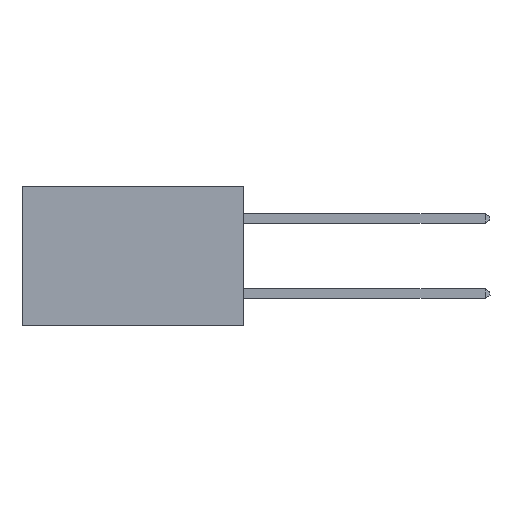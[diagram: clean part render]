
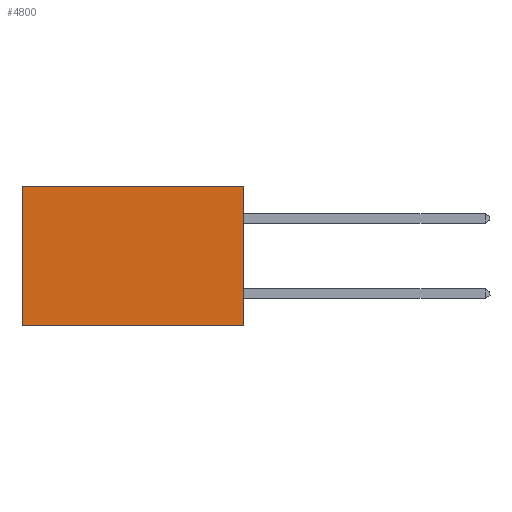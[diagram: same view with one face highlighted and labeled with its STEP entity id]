
A CAD part, left-side view. The second image highlights one B-rep face of the part: STEP entity #4800.
In plain terms, the highlighted planar face has unit normal (-1, 0, 0).
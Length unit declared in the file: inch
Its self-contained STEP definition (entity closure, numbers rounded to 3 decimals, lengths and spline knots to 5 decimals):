
#14 = FACE_OUTER_BOUND ( 'NONE', #2505, .T. ) ;
#333 = ORIENTED_EDGE ( 'NONE', *, *, #8557, .F. ) ;
#865 = EDGE_CURVE ( 'NONE', #5852, #4934, #6939, .T. ) ;
#891 = ORIENTED_EDGE ( 'NONE', *, *, #1129, .T. ) ;
#902 = DIRECTION ( 'NONE',  ( 0., 0., -1. ) ) ;
#1106 = CARTESIAN_POINT ( 'NONE',  ( 0.277, 0.59, -0.37 ) ) ;
#1129 = EDGE_CURVE ( 'NONE', #4934, #6947, #6935, .T. ) ;
#1166 = DIRECTION ( 'NONE',  ( 1., 0., 0. ) ) ;
#1189 = LINE ( 'NONE', #3744, #5350 ) ;
#1469 = CARTESIAN_POINT ( 'NONE',  ( 0.277, 0., -0.37 ) ) ;
#1512 = DIRECTION ( 'NONE',  ( 0., 0., -1. ) ) ;
#1795 = PLANE ( 'NONE',  #5906 ) ;
#2137 = ORIENTED_EDGE ( 'NONE', *, *, #865, .T. ) ;
#2505 = EDGE_LOOP ( 'NONE', ( #891, #333, #3254, #2137 ) ) ;
#3254 = ORIENTED_EDGE ( 'NONE', *, *, #7164, .F. ) ;
#3324 = CARTESIAN_POINT ( 'NONE',  ( 0.277, 0., -0.37 ) ) ;
#3722 = DIRECTION ( 'NONE',  ( 0., 0., -1. ) ) ;
#3744 = CARTESIAN_POINT ( 'NONE',  ( 0.277, 0., -0.37 ) ) ;
#4571 = CARTESIAN_POINT ( 'NONE',  ( 0.277, 0.59, -0.37 ) ) ;
#4641 = VECTOR ( 'NONE', #6700, 39.37008 ) ;
#4800 = ADVANCED_FACE ( 'NONE', ( #14 ), #1795, .F. ) ;
#4934 = VERTEX_POINT ( 'NONE', #7253 ) ;
#5339 = VERTEX_POINT ( 'NONE', #9127 ) ;
#5350 = VECTOR ( 'NONE', #3722, 39.37008 ) ;
#5831 = VECTOR ( 'NONE', #5861, 39.37008 ) ;
#5852 = VERTEX_POINT ( 'NONE', #9854 ) ;
#5861 = DIRECTION ( 'NONE',  ( 0., 1., 0. ) ) ;
#5906 = AXIS2_PLACEMENT_3D ( 'NONE', #1469, #1166, #902 ) ;
#6282 = CARTESIAN_POINT ( 'NONE',  ( 0.277, 0., 0. ) ) ;
#6482 = VECTOR ( 'NONE', #1512, 39.37008 ) ;
#6700 = DIRECTION ( 'NONE',  ( 0., 1., 0. ) ) ;
#6935 = LINE ( 'NONE', #1106, #6482 ) ;
#6939 = LINE ( 'NONE', #6282, #4641 ) ;
#6947 = VERTEX_POINT ( 'NONE', #4571 ) ;
#7164 = EDGE_CURVE ( 'NONE', #5852, #5339, #1189, .T. ) ;
#7253 = CARTESIAN_POINT ( 'NONE',  ( 0.277, 0.59, 0. ) ) ;
#7940 = LINE ( 'NONE', #3324, #5831 ) ;
#8557 = EDGE_CURVE ( 'NONE', #5339, #6947, #7940, .T. ) ;
#9127 = CARTESIAN_POINT ( 'NONE',  ( 0.277, 0., -0.37 ) ) ;
#9854 = CARTESIAN_POINT ( 'NONE',  ( 0.277, 0., 0. ) ) ;
